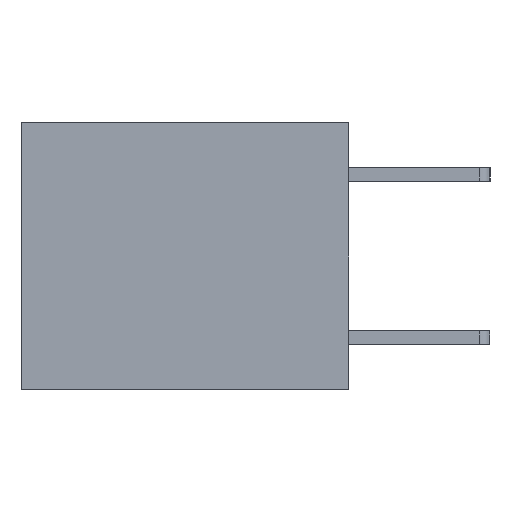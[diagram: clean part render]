
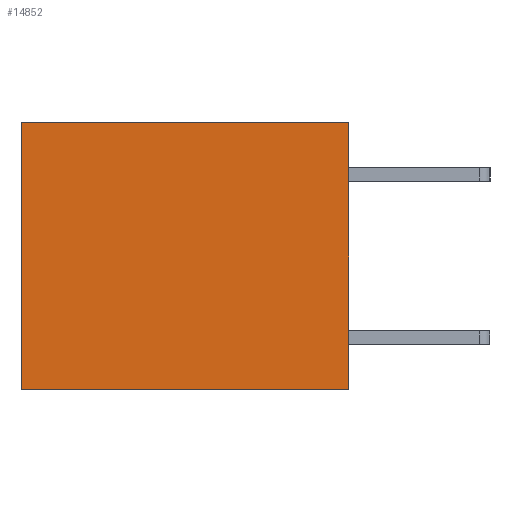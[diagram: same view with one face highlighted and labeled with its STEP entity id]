
A CAD part, left-side view. The second image highlights one B-rep face of the part: STEP entity #14852.
In plain terms, the highlighted planar face has unit normal (-1, 0, 0).
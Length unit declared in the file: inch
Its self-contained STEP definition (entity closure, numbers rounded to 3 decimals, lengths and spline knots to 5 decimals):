
#338 = EDGE_CURVE ( 'NONE', #7556, #5042, #9142, .T. ) ;
#651 = CARTESIAN_POINT ( 'NONE',  ( 0.3165, 0., -0.49 ) ) ;
#1754 = DIRECTION ( 'NONE',  ( 0., 0., -1. ) ) ;
#1987 = LINE ( 'NONE', #11294, #14286 ) ;
#2403 = EDGE_LOOP ( 'NONE', ( #12129, #6539, #14779, #10566 ) ) ;
#2690 = DIRECTION ( 'NONE',  ( 0., 0., -1. ) ) ;
#2753 = VECTOR ( 'NONE', #6271, 39.37008 ) ;
#3373 = CARTESIAN_POINT ( 'NONE',  ( 0.3165, 0.6, -0.49 ) ) ;
#4305 = CARTESIAN_POINT ( 'NONE',  ( 0.3165, 0., 0. ) ) ;
#5042 = VERTEX_POINT ( 'NONE', #651 ) ;
#6271 = DIRECTION ( 'NONE',  ( 0., 1., 0. ) ) ;
#6539 = ORIENTED_EDGE ( 'NONE', *, *, #13558, .F. ) ;
#7556 = VERTEX_POINT ( 'NONE', #4305 ) ;
#7744 = DIRECTION ( 'NONE',  ( 0., 0., -1. ) ) ;
#8948 = AXIS2_PLACEMENT_3D ( 'NONE', #15059, #14845, #7744 ) ;
#9142 = LINE ( 'NONE', #11312, #13804 ) ;
#10566 = ORIENTED_EDGE ( 'NONE', *, *, #10995, .T. ) ;
#10875 = VERTEX_POINT ( 'NONE', #11540 ) ;
#10995 = EDGE_CURVE ( 'NONE', #7556, #10875, #1987, .T. ) ;
#11294 = CARTESIAN_POINT ( 'NONE',  ( 0.3165, 0., 0. ) ) ;
#11312 = CARTESIAN_POINT ( 'NONE',  ( 0.3165, 0., -0.49 ) ) ;
#11521 = PLANE ( 'NONE',  #8948 ) ;
#11540 = CARTESIAN_POINT ( 'NONE',  ( 0.3165, 0.6, 0. ) ) ;
#11607 = EDGE_CURVE ( 'NONE', #10875, #12423, #11705, .T. ) ;
#11705 = LINE ( 'NONE', #14645, #11893 ) ;
#11893 = VECTOR ( 'NONE', #2690, 39.37008 ) ;
#12129 = ORIENTED_EDGE ( 'NONE', *, *, #11607, .T. ) ;
#12423 = VERTEX_POINT ( 'NONE', #3373 ) ;
#12613 = DIRECTION ( 'NONE',  ( 0., 1., 0. ) ) ;
#12803 = LINE ( 'NONE', #13419, #2753 ) ;
#13118 = FACE_OUTER_BOUND ( 'NONE', #2403, .T. ) ;
#13419 = CARTESIAN_POINT ( 'NONE',  ( 0.3165, 0., -0.49 ) ) ;
#13558 = EDGE_CURVE ( 'NONE', #5042, #12423, #12803, .T. ) ;
#13804 = VECTOR ( 'NONE', #1754, 39.37008 ) ;
#14286 = VECTOR ( 'NONE', #12613, 39.37008 ) ;
#14645 = CARTESIAN_POINT ( 'NONE',  ( 0.3165, 0.6, -0.49 ) ) ;
#14779 = ORIENTED_EDGE ( 'NONE', *, *, #338, .F. ) ;
#14845 = DIRECTION ( 'NONE',  ( 1., 0., 0. ) ) ;
#14852 = ADVANCED_FACE ( 'NONE', ( #13118 ), #11521, .F. ) ;
#15059 = CARTESIAN_POINT ( 'NONE',  ( 0.3165, 0., -0.49 ) ) ;
